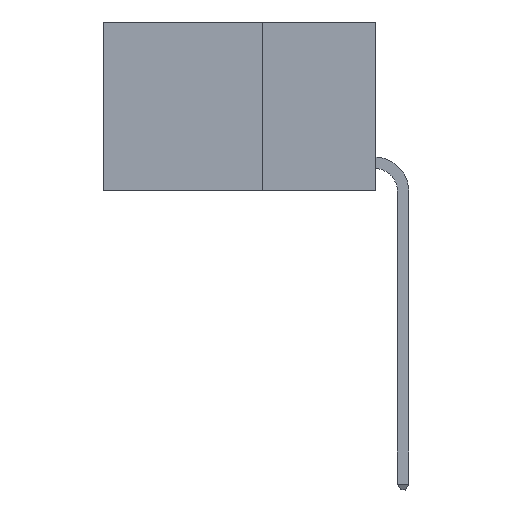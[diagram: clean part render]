
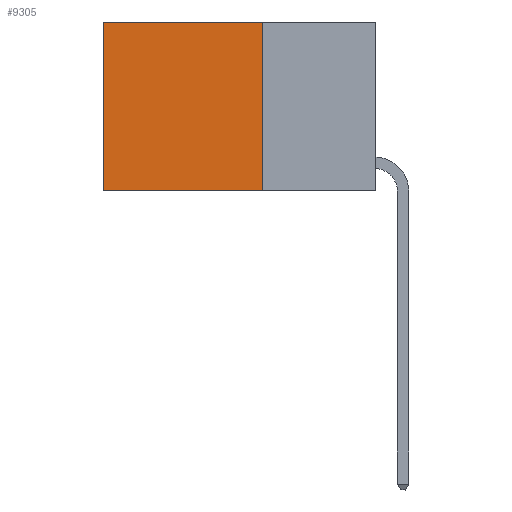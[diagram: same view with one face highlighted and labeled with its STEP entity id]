
A CAD part, left-side view. The second image highlights one B-rep face of the part: STEP entity #9305.
In plain terms, the highlighted planar face has unit normal (-1, 0, 0).
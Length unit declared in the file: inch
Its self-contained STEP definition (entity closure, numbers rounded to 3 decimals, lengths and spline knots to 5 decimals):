
#33 = EDGE_CURVE ( 'NONE', #1344, #3243, #22095, .T. ) ;
#418 = CARTESIAN_POINT ( 'NONE',  ( 0.2625, 0.25, -0.37 ) ) ;
#1344 = VERTEX_POINT ( 'NONE', #418 ) ;
#3243 = VERTEX_POINT ( 'NONE', #14028 ) ;
#3769 = ORIENTED_EDGE ( 'NONE', *, *, #33, .F. ) ;
#3962 = VERTEX_POINT ( 'NONE', #4306 ) ;
#4306 = CARTESIAN_POINT ( 'NONE',  ( 0.2625, 0.25, 0. ) ) ;
#6168 = VECTOR ( 'NONE', #10364, 39.37008 ) ;
#6508 = VERTEX_POINT ( 'NONE', #25697 ) ;
#6756 = EDGE_LOOP ( 'NONE', ( #23081, #3769, #22194, #27466 ) ) ;
#8144 = CARTESIAN_POINT ( 'NONE',  ( 0.2625, 0.6, 0. ) ) ;
#8748 = FACE_OUTER_BOUND ( 'NONE', #6756, .T. ) ;
#9110 = EDGE_CURVE ( 'NONE', #3962, #6508, #19232, .T. ) ;
#9305 = ADVANCED_FACE ( 'NONE', ( #8748 ), #22764, .F. ) ;
#9950 = CARTESIAN_POINT ( 'NONE',  ( 0.2625, 0.25, 0. ) ) ;
#10032 = CARTESIAN_POINT ( 'NONE',  ( 0.2625, 0.25, 0. ) ) ;
#10225 = AXIS2_PLACEMENT_3D ( 'NONE', #9950, #26946, #14315 ) ;
#10364 = DIRECTION ( 'NONE',  ( 0., 0., -1. ) ) ;
#12174 = EDGE_CURVE ( 'NONE', #3962, #1344, #20748, .T. ) ;
#14028 = CARTESIAN_POINT ( 'NONE',  ( 0.2625, 0.6, -0.37 ) ) ;
#14315 = DIRECTION ( 'NONE',  ( 0., 0., -1. ) ) ;
#15066 = VECTOR ( 'NONE', #27023, 39.37008 ) ;
#16454 = VECTOR ( 'NONE', #24407, 39.37008 ) ;
#17486 = CARTESIAN_POINT ( 'NONE',  ( 0.2625, 0.25, 0. ) ) ;
#19232 = LINE ( 'NONE', #17486, #24159 ) ;
#20748 = LINE ( 'NONE', #10032, #15066 ) ;
#21465 = EDGE_CURVE ( 'NONE', #6508, #3243, #23328, .T. ) ;
#22095 = LINE ( 'NONE', #24100, #16454 ) ;
#22194 = ORIENTED_EDGE ( 'NONE', *, *, #12174, .F. ) ;
#22764 = PLANE ( 'NONE',  #10225 ) ;
#23081 = ORIENTED_EDGE ( 'NONE', *, *, #21465, .T. ) ;
#23328 = LINE ( 'NONE', #8144, #6168 ) ;
#23850 = DIRECTION ( 'NONE',  ( 0., 1., 0. ) ) ;
#24100 = CARTESIAN_POINT ( 'NONE',  ( 0.2625, 0.25, -0.37 ) ) ;
#24159 = VECTOR ( 'NONE', #23850, 39.37008 ) ;
#24407 = DIRECTION ( 'NONE',  ( 0., 1., 0. ) ) ;
#25697 = CARTESIAN_POINT ( 'NONE',  ( 0.2625, 0.6, 0. ) ) ;
#26946 = DIRECTION ( 'NONE',  ( 1., 0., 0. ) ) ;
#27023 = DIRECTION ( 'NONE',  ( 0., 0., -1. ) ) ;
#27466 = ORIENTED_EDGE ( 'NONE', *, *, #9110, .T. ) ;
